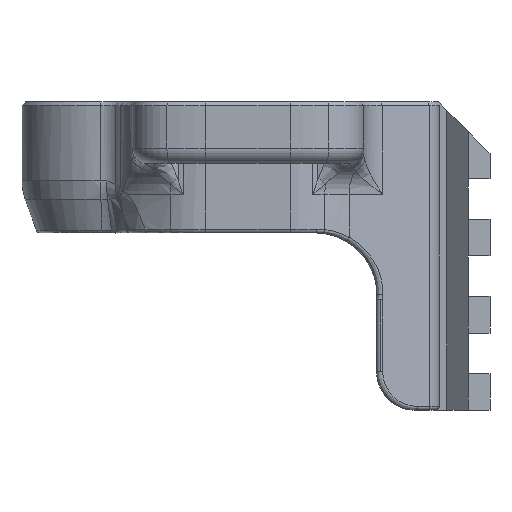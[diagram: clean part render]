
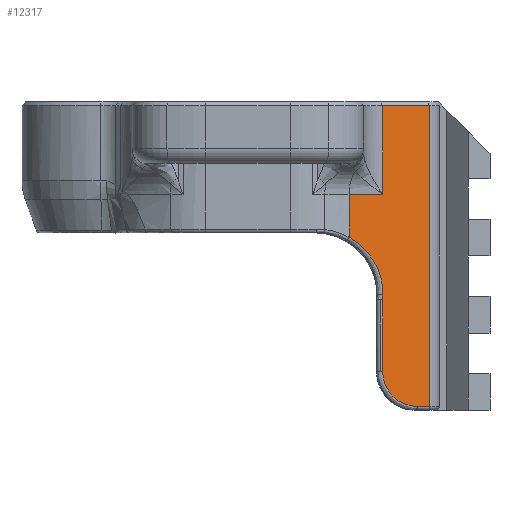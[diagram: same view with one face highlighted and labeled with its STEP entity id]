
A CAD part, left-side view. The second image highlights one B-rep face of the part: STEP entity #12317.
In plain terms, the highlighted planar face has unit normal (-0.808, -0.589, 0).
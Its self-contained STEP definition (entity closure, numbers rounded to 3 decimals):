
#384 = CARTESIAN_POINT ( 'NONE',  ( -14.848, -33.493, -18.679 ) ) ;
#474 = LINE ( 'NONE', #10094, #8693 ) ;
#706 = VECTOR ( 'NONE', #8508, 1000. ) ;
#822 = CARTESIAN_POINT ( 'NONE',  ( -25.642, -18.666, 6.5 ) ) ;
#1270 = FACE_OUTER_BOUND ( 'NONE', #11639, .T. ) ;
#1291 = VERTEX_POINT ( 'NONE', #11685 ) ;
#1298 = CARTESIAN_POINT ( 'NONE',  ( -25.642, -18.666, -32.5 ) ) ;
#1727 = VECTOR ( 'NONE', #11836, 1000. ) ;
#1917 = LINE ( 'NONE', #6971, #5413 ) ;
#1955 = ORIENTED_EDGE ( 'NONE', *, *, #2516, .T. ) ;
#2220 = DIRECTION ( 'NONE',  ( -0.589, 0.808, 0. ) ) ;
#2450 = LINE ( 'NONE', #3465, #6073 ) ;
#2516 = EDGE_CURVE ( 'NONE', #9815, #6695, #3689, .T. ) ;
#2592 = CARTESIAN_POINT ( 'NONE',  ( -14.866, -33.469, -5. ) ) ;
#2730 = CARTESIAN_POINT ( 'NONE',  ( -13.492, -35.357, -32.5 ) ) ;
#2767 = CARTESIAN_POINT ( 'NONE',  ( -18.029, -29.124, -10.562 ) ) ;
#2808 = EDGE_CURVE ( 'NONE', #4571, #1291, #5487, .T. ) ;
#2906 = DIRECTION ( 'NONE',  ( 0., 0., -1. ) ) ;
#3378 = CARTESIAN_POINT ( 'NONE',  ( -14.829, -33.52, -14.83 ) ) ;
#3465 = CARTESIAN_POINT ( 'NONE',  ( -18.029, -29.124, -15. ) ) ;
#3585 = DIRECTION ( 'NONE',  ( 0., 0., 1. ) ) ;
#3689 =( BOUNDED_CURVE ( )  B_SPLINE_CURVE ( 3, ( #7304, #11226, #8400, #7364 ),
 .UNSPECIFIED., .F., .T. ) 
 B_SPLINE_CURVE_WITH_KNOTS ( ( 4, 4 ),
 ( 0., 0.079 ),
 .UNSPECIFIED. ) 
 CURVE ( )  GEOMETRIC_REPRESENTATION_ITEM ( )  RATIONAL_B_SPLINE_CURVE ( ( 1., 0.999, 0.999, 1. ) ) 
 REPRESENTATION_ITEM ( '' )  );
#3771 = EDGE_CURVE ( 'NONE', #4134, #10058, #5483, .T. ) ;
#3812 = CARTESIAN_POINT ( 'NONE',  ( -14.848, -33.493, -30.636 ) ) ;
#3958 = ORIENTED_EDGE ( 'NONE', *, *, #4197, .T. ) ;
#3992 = VERTEX_POINT ( 'NONE', #9783 ) ;
#4134 = VERTEX_POINT ( 'NONE', #8110 ) ;
#4197 = EDGE_CURVE ( 'NONE', #7596, #3992, #474, .T. ) ;
#4206 = VECTOR ( 'NONE', #11237, 1000. ) ;
#4571 = VERTEX_POINT ( 'NONE', #7819 ) ;
#4632 = VECTOR ( 'NONE', #2906, 1000. ) ;
#4681 = ORIENTED_EDGE ( 'NONE', *, *, #8069, .F. ) ;
#4702 = EDGE_CURVE ( 'NONE', #10058, #5270, #6407, .T. ) ;
#5234 = CARTESIAN_POINT ( 'NONE',  ( -18.029, -29.124, -10.562 ) ) ;
#5270 = VERTEX_POINT ( 'NONE', #11525 ) ;
#5344 = CARTESIAN_POINT ( 'NONE',  ( -14.829, -33.52, -18.005 ) ) ;
#5413 = VECTOR ( 'NONE', #12619, 1000. ) ;
#5483 =( BOUNDED_CURVE ( )  B_SPLINE_CURVE ( 3, ( #12473, #3812, #2730, #11504 ),
 .UNSPECIFIED., .F., .T. ) 
 B_SPLINE_CURVE_WITH_KNOTS ( ( 4, 4 ),
 ( 0., 1.571 ),
 .UNSPECIFIED. ) 
 CURVE ( )  GEOMETRIC_REPRESENTATION_ITEM ( )  RATIONAL_B_SPLINE_CURVE ( ( 1., 0.805, 0.805, 1. ) ) 
 REPRESENTATION_ITEM ( '' )  );
#5487 = LINE ( 'NONE', #822, #706 ) ;
#5577 = ORIENTED_EDGE ( 'NONE', *, *, #10314, .T. ) ;
#5735 =( BOUNDED_CURVE ( )  B_SPLINE_CURVE ( 3, ( #5234, #6319, #3378, #5344 ),
 .UNSPECIFIED., .F., .T. ) 
 B_SPLINE_CURVE_WITH_KNOTS ( ( 4, 4 ),
 ( 5.216, 6.283 ),
 .UNSPECIFIED. ) 
 CURVE ( )  GEOMETRIC_REPRESENTATION_ITEM ( )  RATIONAL_B_SPLINE_CURVE ( ( 1., 0.907, 0.907, 1. ) ) 
 REPRESENTATION_ITEM ( '' )  );
#5797 = ORIENTED_EDGE ( 'NONE', *, *, #10563, .T. ) ;
#6073 = VECTOR ( 'NONE', #3585, 1000. ) ;
#6241 = ORIENTED_EDGE ( 'NONE', *, *, #4702, .T. ) ;
#6319 = CARTESIAN_POINT ( 'NONE',  ( -16.005, -31.905, -12.095 ) ) ;
#6321 = DIRECTION ( 'NONE',  ( -0.808, -0.589, 0. ) ) ;
#6407 = LINE ( 'NONE', #1298, #4206 ) ;
#6428 = EDGE_CURVE ( 'NONE', #1291, #7596, #1917, .T. ) ;
#6695 = VERTEX_POINT ( 'NONE', #384 ) ;
#6738 = LINE ( 'NONE', #7703, #4632 ) ;
#6813 = CARTESIAN_POINT ( 'NONE',  ( -10.428, -39.566, -15. ) ) ;
#6971 = CARTESIAN_POINT ( 'NONE',  ( -14.866, -33.469, -1. ) ) ;
#7304 = CARTESIAN_POINT ( 'NONE',  ( -14.829, -33.52, -18.005 ) ) ;
#7364 = CARTESIAN_POINT ( 'NONE',  ( -14.848, -33.493, -18.679 ) ) ;
#7596 = VERTEX_POINT ( 'NONE', #2592 ) ;
#7703 = CARTESIAN_POINT ( 'NONE',  ( -14.848, -33.493, -28. ) ) ;
#7819 = CARTESIAN_POINT ( 'NONE',  ( -10.428, -39.566, 6.5 ) ) ;
#8069 = EDGE_CURVE ( 'NONE', #11333, #3992, #2450, .T. ) ;
#8110 = CARTESIAN_POINT ( 'NONE',  ( -14.848, -33.493, -28. ) ) ;
#8400 = CARTESIAN_POINT ( 'NONE',  ( -14.835, -33.511, -18.455 ) ) ;
#8403 = CARTESIAN_POINT ( 'NONE',  ( -11.573, -37.993, -32.5 ) ) ;
#8417 = CARTESIAN_POINT ( 'NONE',  ( -14.829, -33.52, -18.005 ) ) ;
#8508 = DIRECTION ( 'NONE',  ( -0.589, 0.808, 0. ) ) ;
#8693 = VECTOR ( 'NONE', #2220, 1000. ) ;
#9339 = PLANE ( 'NONE',  #9590 ) ;
#9568 = ORIENTED_EDGE ( 'NONE', *, *, #6428, .T. ) ;
#9590 = AXIS2_PLACEMENT_3D ( 'NONE', #11209, #6321, #11024 ) ;
#9783 = CARTESIAN_POINT ( 'NONE',  ( -18.029, -29.124, -5. ) ) ;
#9815 = VERTEX_POINT ( 'NONE', #8417 ) ;
#9893 = EDGE_CURVE ( 'NONE', #6695, #4134, #6738, .T. ) ;
#10058 = VERTEX_POINT ( 'NONE', #8403 ) ;
#10094 = CARTESIAN_POINT ( 'NONE',  ( -25.642, -18.666, -5. ) ) ;
#10314 = EDGE_CURVE ( 'NONE', #11333, #9815, #5735, .T. ) ;
#10563 = EDGE_CURVE ( 'NONE', #5270, #4571, #11895, .T. ) ;
#11024 = DIRECTION ( 'NONE',  ( -0.589, 0.808, 0. ) ) ;
#11209 = CARTESIAN_POINT ( 'NONE',  ( -25.642, -18.666, -15. ) ) ;
#11226 = CARTESIAN_POINT ( 'NONE',  ( -14.829, -33.52, -18.23 ) ) ;
#11237 = DIRECTION ( 'NONE',  ( 0.589, -0.808, 0. ) ) ;
#11333 = VERTEX_POINT ( 'NONE', #2767 ) ;
#11504 = CARTESIAN_POINT ( 'NONE',  ( -11.573, -37.993, -32.5 ) ) ;
#11525 = CARTESIAN_POINT ( 'NONE',  ( -10.428, -39.566, -32.5 ) ) ;
#11639 = EDGE_LOOP ( 'NONE', ( #4681, #5577, #1955, #12361, #11711, #6241, #5797, #11643, #9568, #3958 ) ) ;
#11643 = ORIENTED_EDGE ( 'NONE', *, *, #2808, .T. ) ;
#11685 = CARTESIAN_POINT ( 'NONE',  ( -14.866, -33.469, 6.5 ) ) ;
#11711 = ORIENTED_EDGE ( 'NONE', *, *, #3771, .T. ) ;
#11836 = DIRECTION ( 'NONE',  ( 0., 0., 1. ) ) ;
#11895 = LINE ( 'NONE', #6813, #1727 ) ;
#12317 = ADVANCED_FACE ( 'NONE', ( #1270 ), #9339, .T. ) ;
#12361 = ORIENTED_EDGE ( 'NONE', *, *, #9893, .T. ) ;
#12473 = CARTESIAN_POINT ( 'NONE',  ( -14.848, -33.493, -28. ) ) ;
#12619 = DIRECTION ( 'NONE',  ( 0., 0., -1. ) ) ;
